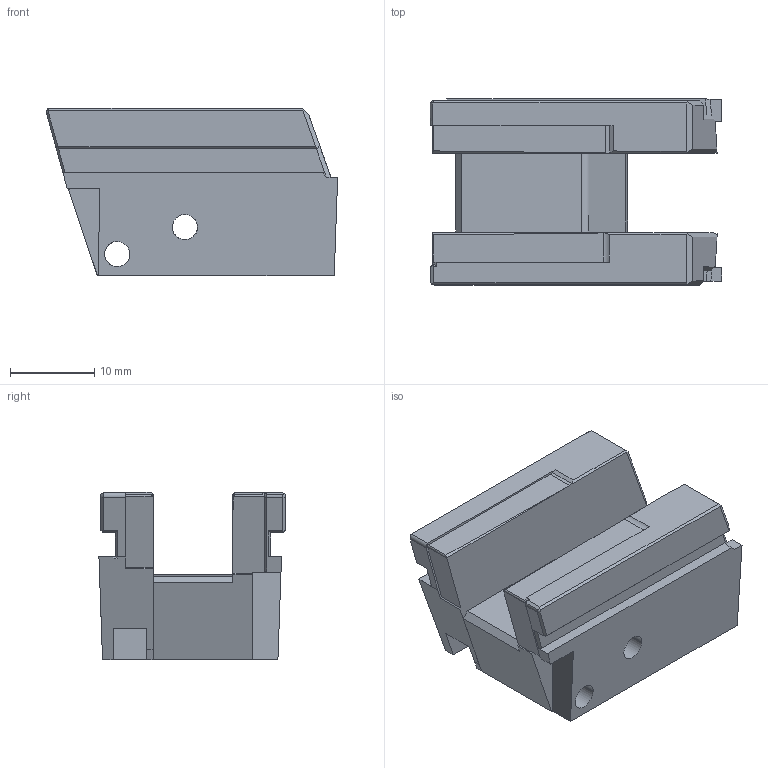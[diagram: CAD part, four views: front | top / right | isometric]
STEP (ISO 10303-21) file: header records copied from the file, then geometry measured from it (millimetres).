
FILE_DESCRIPTION (( 'STEP AP214' ), '1' );
FILE_NAME ('3089 Rear Rail Block.STEP', '2022-08-18T01:02:16', ( '' ), ( '' ), 'SwSTEP 2.0', 'SolidWorks 2020', '' );
FILE_SCHEMA (( 'AUTOMOTIVE_DESIGN' ));
Length unit declared in the file: millimetre
Products named in the file (1): 3089 Rear Rail Block
Bounding box: 34.65 x 22.14 x 19.87 mm (x, y, z)
Volume: 7992.3 mm3; surface area: 4382.2 mm2
Topology: 1 solids, 1 shells, 130 faces, 380 edges, 250 vertices
Faces by surface type: plane 105, cylinder 14, bspline 6, cone 5
Entity records: 4660 total; most frequent: CARTESIAN_POINT 1482, ORIENTED_EDGE 760, DIRECTION 501, EDGE_CURVE 380, VERTEX_POINT 250, LINE 217, VECTOR 217, AXIS2_PLACEMENT_3D 142
